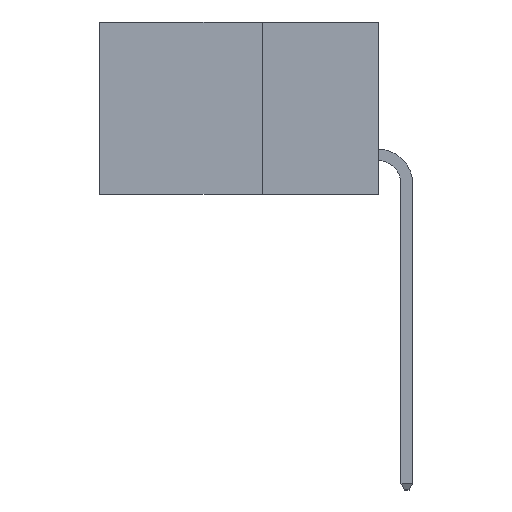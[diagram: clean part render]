
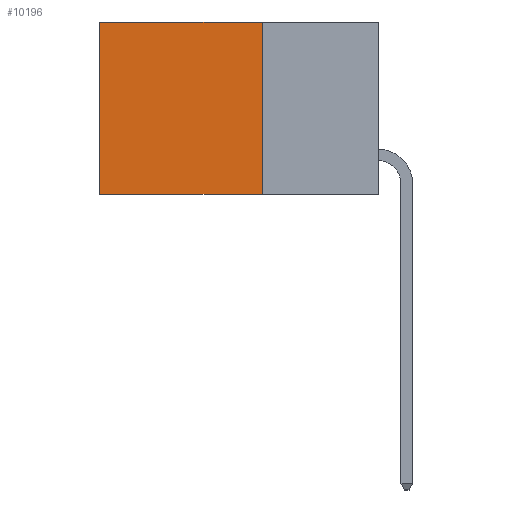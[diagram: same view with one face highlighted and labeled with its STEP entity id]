
A CAD part, left-side view. The second image highlights one B-rep face of the part: STEP entity #10196.
In plain terms, the highlighted planar face has unit normal (-1, 0, 0).
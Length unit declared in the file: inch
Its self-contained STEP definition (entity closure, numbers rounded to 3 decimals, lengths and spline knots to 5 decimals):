
#35 = CARTESIAN_POINT ( 'NONE',  ( 0.2615, 0.25, 0. ) ) ;
#390 = DIRECTION ( 'NONE',  ( 0., 0., -1. ) ) ;
#731 = VECTOR ( 'NONE', #6299, 39.37008 ) ;
#732 = ORIENTED_EDGE ( 'NONE', *, *, #4717, .F. ) ;
#741 = FACE_OUTER_BOUND ( 'NONE', #10107, .T. ) ;
#1120 = AXIS2_PLACEMENT_3D ( 'NONE', #8186, #5976, #11600 ) ;
#1406 = CARTESIAN_POINT ( 'NONE',  ( 0.2615, 0.6, 0. ) ) ;
#2168 = LINE ( 'NONE', #35, #7142 ) ;
#2323 = CARTESIAN_POINT ( 'NONE',  ( 0.2615, 0.25, -0.37 ) ) ;
#2412 = CARTESIAN_POINT ( 'NONE',  ( 0.2615, 0.25, 0. ) ) ;
#2826 = ORIENTED_EDGE ( 'NONE', *, *, #13167, .T. ) ;
#2937 = EDGE_CURVE ( 'NONE', #9542, #13749, #3251, .T. ) ;
#2949 = CARTESIAN_POINT ( 'NONE',  ( 0.2615, 0.6, -0.37 ) ) ;
#3251 = LINE ( 'NONE', #2323, #4952 ) ;
#4213 = LINE ( 'NONE', #4513, #11579 ) ;
#4513 = CARTESIAN_POINT ( 'NONE',  ( 0.2615, 0.25, -0.37 ) ) ;
#4717 = EDGE_CURVE ( 'NONE', #6074, #9542, #4213, .T. ) ;
#4952 = VECTOR ( 'NONE', #9964, 39.37008 ) ;
#5711 = LINE ( 'NONE', #2949, #731 ) ;
#5976 = DIRECTION ( 'NONE',  ( 1., 0., 0. ) ) ;
#6074 = VERTEX_POINT ( 'NONE', #2412 ) ;
#6299 = DIRECTION ( 'NONE',  ( 0., 0., -1. ) ) ;
#6546 = DIRECTION ( 'NONE',  ( 0., 1., 0. ) ) ;
#7142 = VECTOR ( 'NONE', #6546, 39.37008 ) ;
#7598 = CARTESIAN_POINT ( 'NONE',  ( 0.2615, 0.25, -0.37 ) ) ;
#8186 = CARTESIAN_POINT ( 'NONE',  ( 0.2615, 0.25, -0.37 ) ) ;
#9542 = VERTEX_POINT ( 'NONE', #7598 ) ;
#9964 = DIRECTION ( 'NONE',  ( 0., 1., 0. ) ) ;
#10107 = EDGE_LOOP ( 'NONE', ( #11720, #13609, #732, #2826 ) ) ;
#10196 = ADVANCED_FACE ( 'NONE', ( #741 ), #12292, .F. ) ;
#10302 = EDGE_CURVE ( 'NONE', #11706, #13749, #5711, .T. ) ;
#11060 = CARTESIAN_POINT ( 'NONE',  ( 0.2615, 0.6, -0.37 ) ) ;
#11579 = VECTOR ( 'NONE', #390, 39.37008 ) ;
#11600 = DIRECTION ( 'NONE',  ( 0., 0., -1. ) ) ;
#11706 = VERTEX_POINT ( 'NONE', #1406 ) ;
#11720 = ORIENTED_EDGE ( 'NONE', *, *, #10302, .T. ) ;
#12292 = PLANE ( 'NONE',  #1120 ) ;
#13167 = EDGE_CURVE ( 'NONE', #6074, #11706, #2168, .T. ) ;
#13609 = ORIENTED_EDGE ( 'NONE', *, *, #2937, .F. ) ;
#13749 = VERTEX_POINT ( 'NONE', #11060 ) ;
